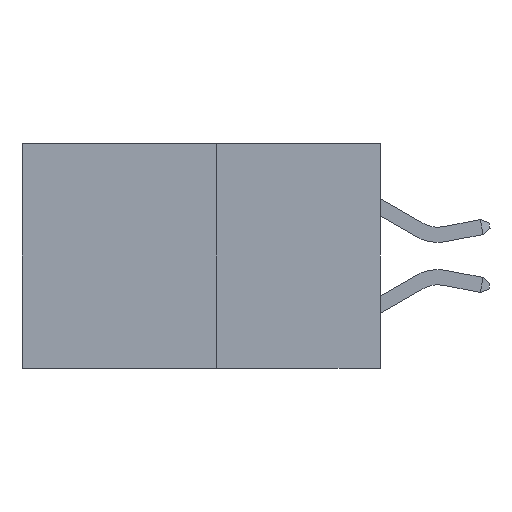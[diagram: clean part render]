
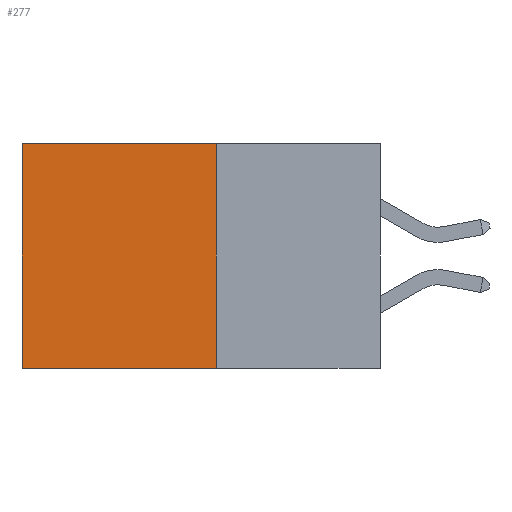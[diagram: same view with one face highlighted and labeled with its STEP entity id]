
A CAD part, left-side view. The second image highlights one B-rep face of the part: STEP entity #277.
In plain terms, the highlighted planar face has unit normal (-1, 0, 0).
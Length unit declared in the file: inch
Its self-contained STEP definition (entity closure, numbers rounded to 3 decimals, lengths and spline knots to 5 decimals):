
#277 = ADVANCED_FACE ( 'NONE', ( #7561 ), #3728, .F. ) ;
#384 = EDGE_CURVE ( 'NONE', #438, #1977, #607, .T. ) ;
#438 = VERTEX_POINT ( 'NONE', #5451 ) ;
#517 = ORIENTED_EDGE ( 'NONE', *, *, #384, .F. ) ;
#607 = LINE ( 'NONE', #5354, #2513 ) ;
#1569 = CARTESIAN_POINT ( 'NONE',  ( 0.277, 0.27, -0.37 ) ) ;
#1596 = EDGE_LOOP ( 'NONE', ( #9009, #4132, #517, #3911 ) ) ;
#1632 = CARTESIAN_POINT ( 'NONE',  ( 0.277, 0.27, -0.37 ) ) ;
#1715 = VERTEX_POINT ( 'NONE', #7161 ) ;
#1977 = VERTEX_POINT ( 'NONE', #1569 ) ;
#2513 = VECTOR ( 'NONE', #4379, 39.37008 ) ;
#2935 = CARTESIAN_POINT ( 'NONE',  ( 0.277, 0.27, -0.37 ) ) ;
#3463 = DIRECTION ( 'NONE',  ( 1., 0., 0. ) ) ;
#3728 = PLANE ( 'NONE',  #6727 ) ;
#3911 = ORIENTED_EDGE ( 'NONE', *, *, #6896, .T. ) ;
#3924 = DIRECTION ( 'NONE',  ( 0., 0., -1. ) ) ;
#4132 = ORIENTED_EDGE ( 'NONE', *, *, #7238, .F. ) ;
#4379 = DIRECTION ( 'NONE',  ( 0., 0., -1. ) ) ;
#4593 = CARTESIAN_POINT ( 'NONE',  ( 0.277, 0.27, 0. ) ) ;
#4708 = CARTESIAN_POINT ( 'NONE',  ( 0.277, 0.59, 0. ) ) ;
#4771 = VERTEX_POINT ( 'NONE', #4708 ) ;
#4903 = VECTOR ( 'NONE', #6343, 39.37008 ) ;
#5354 = CARTESIAN_POINT ( 'NONE',  ( 0.277, 0.27, -0.37 ) ) ;
#5451 = CARTESIAN_POINT ( 'NONE',  ( 0.277, 0.27, 0. ) ) ;
#6343 = DIRECTION ( 'NONE',  ( 0., 1., 0. ) ) ;
#6461 = CARTESIAN_POINT ( 'NONE',  ( 0.277, 0.59, -0.37 ) ) ;
#6589 = DIRECTION ( 'NONE',  ( 0., 0., -1. ) ) ;
#6667 = DIRECTION ( 'NONE',  ( 0., 1., 0. ) ) ;
#6727 = AXIS2_PLACEMENT_3D ( 'NONE', #2935, #3463, #3924 ) ;
#6896 = EDGE_CURVE ( 'NONE', #438, #4771, #7155, .T. ) ;
#7155 = LINE ( 'NONE', #4593, #4903 ) ;
#7161 = CARTESIAN_POINT ( 'NONE',  ( 0.277, 0.59, -0.37 ) ) ;
#7238 = EDGE_CURVE ( 'NONE', #1977, #1715, #7943, .T. ) ;
#7528 = LINE ( 'NONE', #6461, #8615 ) ;
#7561 = FACE_OUTER_BOUND ( 'NONE', #1596, .T. ) ;
#7739 = VECTOR ( 'NONE', #6667, 39.37008 ) ;
#7943 = LINE ( 'NONE', #1632, #7739 ) ;
#8615 = VECTOR ( 'NONE', #6589, 39.37008 ) ;
#8995 = EDGE_CURVE ( 'NONE', #4771, #1715, #7528, .T. ) ;
#9009 = ORIENTED_EDGE ( 'NONE', *, *, #8995, .T. ) ;
